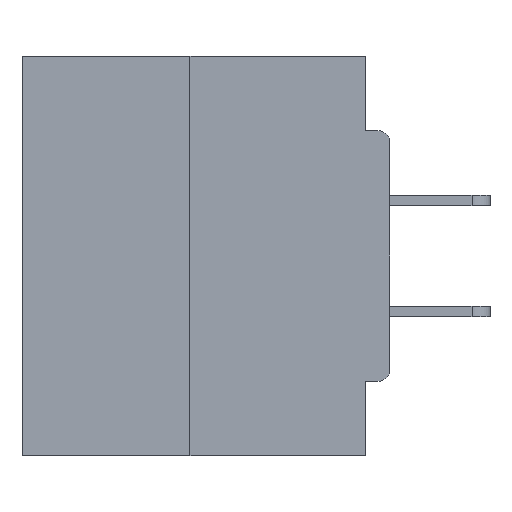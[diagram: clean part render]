
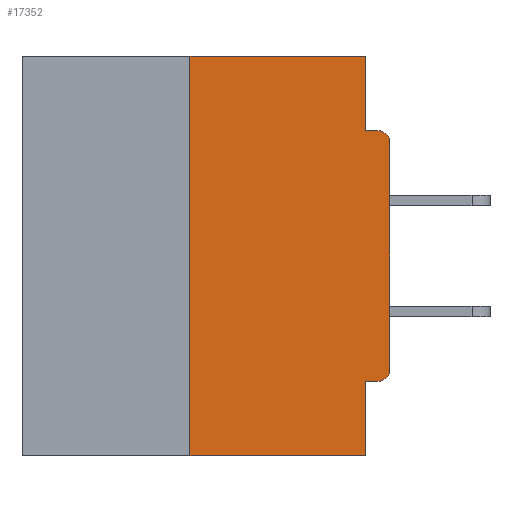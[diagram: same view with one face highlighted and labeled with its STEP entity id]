
A CAD part, left-side view. The second image highlights one B-rep face of the part: STEP entity #17352.
In plain terms, the highlighted planar face has unit normal (-1, 0, 0).
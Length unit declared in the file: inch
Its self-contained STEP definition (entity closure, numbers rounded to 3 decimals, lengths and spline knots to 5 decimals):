
#367 = CARTESIAN_POINT ( 'NONE',  ( 0., 0., -0.0935 ) ) ;
#681 = VERTEX_POINT ( 'NONE', #4357 ) ;
#884 = EDGE_CURVE ( 'NONE', #16656, #20363, #8572, .T. ) ;
#896 = CARTESIAN_POINT ( 'NONE',  ( 0., 0.46, -0.5 ) ) ;
#1111 = ORIENTED_EDGE ( 'NONE', *, *, #2230, .T. ) ;
#1977 = VERTEX_POINT ( 'NONE', #12188 ) ;
#2230 = EDGE_CURVE ( 'NONE', #28134, #19500, #11016, .T. ) ;
#2638 = DIRECTION ( 'NONE',  ( 0., -1., 0. ) ) ;
#3038 = DIRECTION ( 'NONE',  ( 0., -1., 0. ) ) ;
#3194 = CARTESIAN_POINT ( 'NONE',  ( 0., 0., -0.3915 ) ) ;
#3326 = DIRECTION ( 'NONE',  ( 0., -1., 0. ) ) ;
#3955 = EDGE_LOOP ( 'NONE', ( #26992, #16390, #32577, #12090, #8424, #1111, #17748, #13554, #4259, #33785 ) ) ;
#4259 = ORIENTED_EDGE ( 'NONE', *, *, #26844, .F. ) ;
#4357 = CARTESIAN_POINT ( 'NONE',  ( 0., 0.031, -0.0935 ) ) ;
#4508 = PLANE ( 'NONE',  #6402 ) ;
#4883 = EDGE_CURVE ( 'NONE', #20363, #681, #22126, .T. ) ;
#5154 = VERTEX_POINT ( 'NONE', #27261 ) ;
#5487 = CARTESIAN_POINT ( 'NONE',  ( 0., 0.25, 0. ) ) ;
#5860 = LINE ( 'NONE', #367, #10610 ) ;
#6026 = VERTEX_POINT ( 'NONE', #22375 ) ;
#6327 = AXIS2_PLACEMENT_3D ( 'NONE', #30060, #13604, #30539 ) ;
#6402 = AXIS2_PLACEMENT_3D ( 'NONE', #15651, #35250, #18567 ) ;
#7202 = LINE ( 'NONE', #20201, #27665 ) ;
#8184 = LINE ( 'NONE', #23134, #30808 ) ;
#8424 = ORIENTED_EDGE ( 'NONE', *, *, #15103, .F. ) ;
#8550 = FACE_OUTER_BOUND ( 'NONE', #3955, .T. ) ;
#8572 = LINE ( 'NONE', #19254, #28608 ) ;
#10174 = CARTESIAN_POINT ( 'NONE',  ( 0., 0.031, -0.4065 ) ) ;
#10610 = VECTOR ( 'NONE', #3038, 39.37008 ) ;
#10937 = DIRECTION ( 'NONE',  ( 0., 0., 1. ) ) ;
#11016 = CIRCLE ( 'NONE', #6327, 0.015 ) ;
#11052 = EDGE_CURVE ( 'NONE', #13310, #29922, #30211, .T. ) ;
#11244 = VECTOR ( 'NONE', #31448, 39.37008 ) ;
#11939 = CARTESIAN_POINT ( 'NONE',  ( 0., 0.031, -0.5 ) ) ;
#12090 = ORIENTED_EDGE ( 'NONE', *, *, #11052, .F. ) ;
#12188 = CARTESIAN_POINT ( 'NONE',  ( 0., 0.25, -0.5 ) ) ;
#12442 = LINE ( 'NONE', #896, #22912 ) ;
#13310 = VERTEX_POINT ( 'NONE', #10174 ) ;
#13554 = ORIENTED_EDGE ( 'NONE', *, *, #32906, .T. ) ;
#13604 = DIRECTION ( 'NONE',  ( -1., 0., 0. ) ) ;
#14184 = VECTOR ( 'NONE', #10937, 39.37008 ) ;
#14959 = DIRECTION ( 'NONE',  ( 0., 1., 0. ) ) ;
#15025 = DIRECTION ( 'NONE',  ( 0., 0., -1. ) ) ;
#15103 = EDGE_CURVE ( 'NONE', #28134, #13310, #7202, .T. ) ;
#15217 = DIRECTION ( 'NONE',  ( 0., 0., 1. ) ) ;
#15651 = CARTESIAN_POINT ( 'NONE',  ( 0., 0.46, 0. ) ) ;
#15793 = VECTOR ( 'NONE', #15025, 39.37008 ) ;
#16390 = ORIENTED_EDGE ( 'NONE', *, *, #25608, .F. ) ;
#16656 = VERTEX_POINT ( 'NONE', #19763 ) ;
#17172 = AXIS2_PLACEMENT_3D ( 'NONE', #27482, #19065, #24678 ) ;
#17314 = EDGE_CURVE ( 'NONE', #1977, #29922, #12442, .T. ) ;
#17352 = ADVANCED_FACE ( 'NONE', ( #8550 ), #4508, .F. ) ;
#17748 = ORIENTED_EDGE ( 'NONE', *, *, #24115, .T. ) ;
#18567 = DIRECTION ( 'NONE',  ( 0., 0., -1. ) ) ;
#19053 = CARTESIAN_POINT ( 'NONE',  ( 0., 0.015, -0.4065 ) ) ;
#19065 = DIRECTION ( 'NONE',  ( -1., 0., 0. ) ) ;
#19254 = CARTESIAN_POINT ( 'NONE',  ( 0., 0.46, 0. ) ) ;
#19500 = VERTEX_POINT ( 'NONE', #3194 ) ;
#19508 = CARTESIAN_POINT ( 'NONE',  ( 0., 0.031, 0. ) ) ;
#19763 = CARTESIAN_POINT ( 'NONE',  ( 0., 0.25, 0. ) ) ;
#19821 = CIRCLE ( 'NONE', #17172, 0.015 ) ;
#20000 = CARTESIAN_POINT ( 'NONE',  ( 0., 0.031, 0. ) ) ;
#20201 = CARTESIAN_POINT ( 'NONE',  ( 0., 0., -0.4065 ) ) ;
#20363 = VERTEX_POINT ( 'NONE', #19508 ) ;
#22126 = LINE ( 'NONE', #20000, #11244 ) ;
#22375 = CARTESIAN_POINT ( 'NONE',  ( 0., 0.015, -0.0935 ) ) ;
#22912 = VECTOR ( 'NONE', #3326, 39.37008 ) ;
#23134 = CARTESIAN_POINT ( 'NONE',  ( 0., 0., 0. ) ) ;
#23297 = CARTESIAN_POINT ( 'NONE',  ( 0., 0.031, -0.5 ) ) ;
#24115 = EDGE_CURVE ( 'NONE', #19500, #5154, #8184, .T. ) ;
#24678 = DIRECTION ( 'NONE',  ( 0., 0., -1. ) ) ;
#25608 = EDGE_CURVE ( 'NONE', #1977, #16656, #31611, .T. ) ;
#26844 = EDGE_CURVE ( 'NONE', #681, #6026, #5860, .T. ) ;
#26992 = ORIENTED_EDGE ( 'NONE', *, *, #884, .F. ) ;
#27261 = CARTESIAN_POINT ( 'NONE',  ( 0., 0., -0.1085 ) ) ;
#27482 = CARTESIAN_POINT ( 'NONE',  ( 0., 0.015, -0.1085 ) ) ;
#27665 = VECTOR ( 'NONE', #14959, 39.37008 ) ;
#28134 = VERTEX_POINT ( 'NONE', #19053 ) ;
#28608 = VECTOR ( 'NONE', #2638, 39.37008 ) ;
#29922 = VERTEX_POINT ( 'NONE', #11939 ) ;
#30060 = CARTESIAN_POINT ( 'NONE',  ( 0., 0.015, -0.3915 ) ) ;
#30211 = LINE ( 'NONE', #23297, #15793 ) ;
#30539 = DIRECTION ( 'NONE',  ( 0., 0., -1. ) ) ;
#30808 = VECTOR ( 'NONE', #15217, 39.37008 ) ;
#31448 = DIRECTION ( 'NONE',  ( 0., 0., -1. ) ) ;
#31611 = LINE ( 'NONE', #5487, #14184 ) ;
#32577 = ORIENTED_EDGE ( 'NONE', *, *, #17314, .T. ) ;
#32906 = EDGE_CURVE ( 'NONE', #5154, #6026, #19821, .T. ) ;
#33785 = ORIENTED_EDGE ( 'NONE', *, *, #4883, .F. ) ;
#35250 = DIRECTION ( 'NONE',  ( 1., 0., 0. ) ) ;
